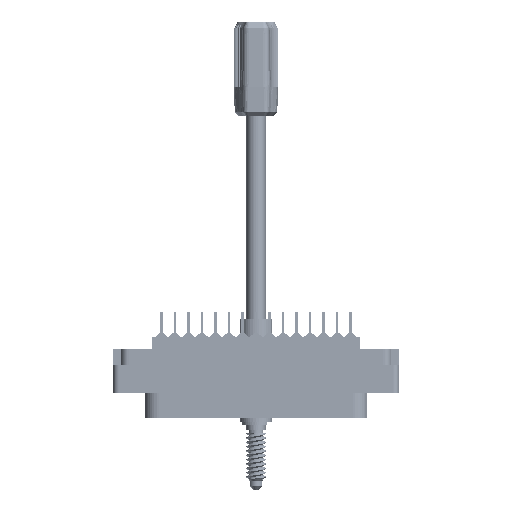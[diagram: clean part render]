
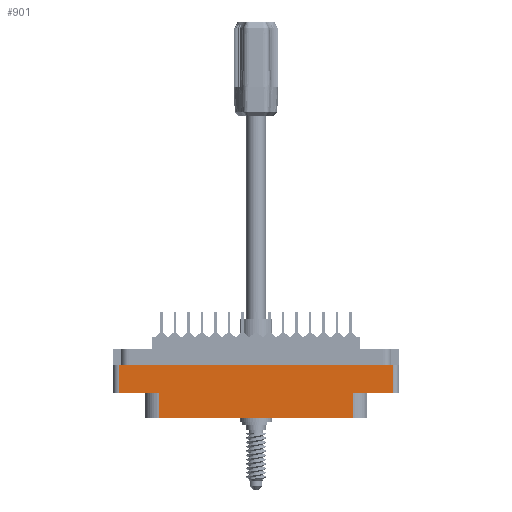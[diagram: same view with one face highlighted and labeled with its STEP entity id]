
A CAD part, front view. The second image highlights one B-rep face of the part: STEP entity #901.
In plain terms, the highlighted planar face has unit normal (0, -1, 0).
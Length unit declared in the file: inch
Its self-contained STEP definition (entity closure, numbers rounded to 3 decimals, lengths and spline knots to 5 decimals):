
#366 = EDGE_CURVE ( 'NONE', #37949, #74454, #82910, .T. ) ;
#901 = ADVANCED_FACE ( 'NONE', ( #95268 ), #59210, .T. ) ;
#1820 = CARTESIAN_POINT ( 'NONE',  ( -1.375, -0.7625, -0.78 ) ) ;
#2579 = CARTESIAN_POINT ( 'NONE',  ( 0.9315, -0.7625, -0.54 ) ) ;
#2634 = CARTESIAN_POINT ( 'NONE',  ( 1.313, -0.7625, -0.54 ) ) ;
#2984 = CARTESIAN_POINT ( 'NONE',  ( -1.313, -0.7625, -0.54 ) ) ;
#7596 = LINE ( 'NONE', #58622, #68721 ) ;
#12456 = CARTESIAN_POINT ( 'NONE',  ( -1.375, -0.7625, -0.78 ) ) ;
#13851 = ORIENTED_EDGE ( 'NONE', *, *, #98295, .T. ) ;
#14052 = DIRECTION ( 'NONE',  ( -1., 0., 0. ) ) ;
#17970 = CARTESIAN_POINT ( 'NONE',  ( -1.313, -0.7625, -0.274 ) ) ;
#18566 = DIRECTION ( 'NONE',  ( 0., 0., 1. ) ) ;
#20472 = EDGE_CURVE ( 'NONE', #68672, #64658, #75390, .T. ) ;
#24049 = ORIENTED_EDGE ( 'NONE', *, *, #39654, .T. ) ;
#26349 = CARTESIAN_POINT ( 'NONE',  ( 0.9315, -0.7625, -0.54 ) ) ;
#26998 = ORIENTED_EDGE ( 'NONE', *, *, #20472, .T. ) ;
#28555 = DIRECTION ( 'NONE',  ( 0., -1., 0. ) ) ;
#31779 = VECTOR ( 'NONE', #14052, 39.37008 ) ;
#33968 = DIRECTION ( 'NONE',  ( 1., 0., 0. ) ) ;
#34716 = EDGE_CURVE ( 'NONE', #68672, #39679, #61158, .T. ) ;
#35671 = EDGE_LOOP ( 'NONE', ( #58388, #26998, #24049, #83284, #73235, #42825, #59014, #13851 ) ) ;
#37618 = DIRECTION ( 'NONE',  ( 0., 0., 1. ) ) ;
#37949 = VERTEX_POINT ( 'NONE', #2634 ) ;
#38278 = EDGE_CURVE ( 'NONE', #97711, #57576, #101537, .T. ) ;
#39654 = EDGE_CURVE ( 'NONE', #64658, #97711, #7596, .T. ) ;
#39679 = VERTEX_POINT ( 'NONE', #82113 ) ;
#41958 = VECTOR ( 'NONE', #37618, 39.37008 ) ;
#42825 = ORIENTED_EDGE ( 'NONE', *, *, #87712, .T. ) ;
#44405 = VERTEX_POINT ( 'NONE', #63741 ) ;
#44980 = VECTOR ( 'NONE', #45652, 39.37008 ) ;
#45652 = DIRECTION ( 'NONE',  ( 1., 0., 0. ) ) ;
#45765 = CARTESIAN_POINT ( 'NONE',  ( -0.9315, -0.7625, -0.54 ) ) ;
#46546 = VECTOR ( 'NONE', #86736, 39.37008 ) ;
#46880 = CARTESIAN_POINT ( 'NONE',  ( -0.9315, -0.7625, -0.78 ) ) ;
#47662 = LINE ( 'NONE', #2579, #102677 ) ;
#52587 = DIRECTION ( 'NONE',  ( 0., 0., -1. ) ) ;
#57576 = VERTEX_POINT ( 'NONE', #64443 ) ;
#58388 = ORIENTED_EDGE ( 'NONE', *, *, #34716, .F. ) ;
#58622 = CARTESIAN_POINT ( 'NONE',  ( 0., -0.7625, -0.54 ) ) ;
#59014 = ORIENTED_EDGE ( 'NONE', *, *, #366, .F. ) ;
#59210 = PLANE ( 'NONE',  #83882 ) ;
#60346 = LINE ( 'NONE', #1820, #62881 ) ;
#61158 = LINE ( 'NONE', #100809, #44980 ) ;
#62881 = VECTOR ( 'NONE', #96062, 39.37008 ) ;
#63741 = CARTESIAN_POINT ( 'NONE',  ( 0.9315, -0.7625, -0.78 ) ) ;
#64443 = CARTESIAN_POINT ( 'NONE',  ( -0.9315, -0.7625, -0.78 ) ) ;
#64658 = VERTEX_POINT ( 'NONE', #2984 ) ;
#68672 = VERTEX_POINT ( 'NONE', #17970 ) ;
#68721 = VECTOR ( 'NONE', #33968, 39.37008 ) ;
#70101 = DIRECTION ( 'NONE',  ( 0., 0., -1. ) ) ;
#71132 = CARTESIAN_POINT ( 'NONE',  ( -1.313, -0.7625, -0.78 ) ) ;
#71239 = CARTESIAN_POINT ( 'NONE',  ( 0., -0.7625, -0.54 ) ) ;
#71502 = LINE ( 'NONE', #77354, #41958 ) ;
#73235 = ORIENTED_EDGE ( 'NONE', *, *, #86571, .T. ) ;
#74454 = VERTEX_POINT ( 'NONE', #26349 ) ;
#75390 = LINE ( 'NONE', #71132, #82990 ) ;
#77354 = CARTESIAN_POINT ( 'NONE',  ( 1.313, -0.7625, -0.78 ) ) ;
#82113 = CARTESIAN_POINT ( 'NONE',  ( 1.313, -0.7625, -0.274 ) ) ;
#82910 = LINE ( 'NONE', #71239, #31779 ) ;
#82990 = VECTOR ( 'NONE', #70101, 39.37008 ) ;
#83284 = ORIENTED_EDGE ( 'NONE', *, *, #38278, .T. ) ;
#83882 = AXIS2_PLACEMENT_3D ( 'NONE', #12456, #28555, #52587 ) ;
#86571 = EDGE_CURVE ( 'NONE', #57576, #44405, #60346, .T. ) ;
#86736 = DIRECTION ( 'NONE',  ( 0., 0., -1. ) ) ;
#87712 = EDGE_CURVE ( 'NONE', #44405, #74454, #47662, .T. ) ;
#95268 = FACE_OUTER_BOUND ( 'NONE', #35671, .T. ) ;
#96062 = DIRECTION ( 'NONE',  ( 1., 0., 0. ) ) ;
#97711 = VERTEX_POINT ( 'NONE', #45765 ) ;
#98295 = EDGE_CURVE ( 'NONE', #37949, #39679, #71502, .T. ) ;
#100809 = CARTESIAN_POINT ( 'NONE',  ( 0., -0.7625, -0.274 ) ) ;
#101537 = LINE ( 'NONE', #46880, #46546 ) ;
#102677 = VECTOR ( 'NONE', #18566, 39.37008 ) ;
